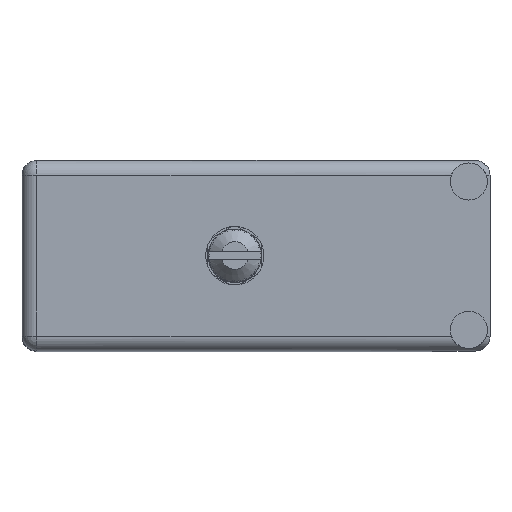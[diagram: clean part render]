
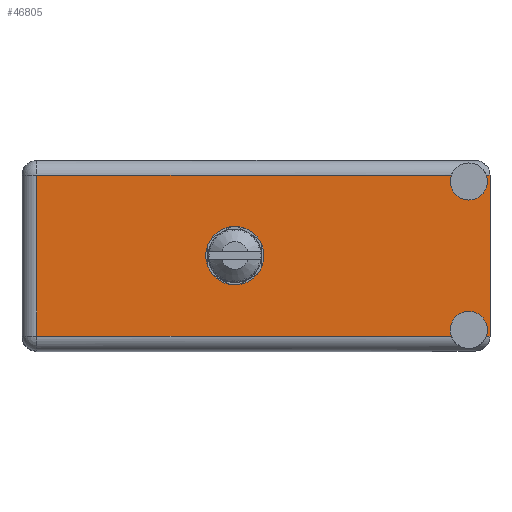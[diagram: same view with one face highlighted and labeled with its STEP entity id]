
A CAD part, top view. The second image highlights one B-rep face of the part: STEP entity #46805.
In plain terms, the highlighted face is planar.
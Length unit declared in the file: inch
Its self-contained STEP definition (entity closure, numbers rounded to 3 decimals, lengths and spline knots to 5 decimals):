
#217 = EDGE_CURVE ( 'NONE', #81219, #66211, #25588, .T. ) ;
#3424 = CARTESIAN_POINT ( 'NONE',  ( 2.19038, 1.566, -0.829 ) ) ;
#3814 = DIRECTION ( 'NONE',  ( 0., 1., 0. ) ) ;
#3861 = LINE ( 'NONE', #11633, #55414 ) ;
#5197 = CARTESIAN_POINT ( 'NONE',  ( 2.108, 1.566, -0.7995 ) ) ;
#6109 = CARTESIAN_POINT ( 'NONE',  ( 2.108, 1.566, -0.0995 ) ) ;
#7385 = AXIS2_PLACEMENT_3D ( 'NONE', #73167, #33031, #65398 ) ;
#7603 = VERTEX_POINT ( 'NONE', #69395 ) ;
#9852 = AXIS2_PLACEMENT_3D ( 'NONE', #26277, #73472, #17136 ) ;
#10412 = EDGE_CURVE ( 'NONE', #15194, #74606, #84376, .T. ) ;
#10895 = LINE ( 'NONE', #34693, #63753 ) ;
#11633 = CARTESIAN_POINT ( 'NONE',  ( 0., 1.566, -0.829 ) ) ;
#12533 = CARTESIAN_POINT ( 'NONE',  ( 0., 1.566, -0.829 ) ) ;
#14298 = CARTESIAN_POINT ( 'NONE',  ( 0.07, 1.566, -0.07 ) ) ;
#14692 = DIRECTION ( 'NONE',  ( 1., 0., 0. ) ) ;
#14764 = VERTEX_POINT ( 'NONE', #14298 ) ;
#15009 = ORIENTED_EDGE ( 'NONE', *, *, #86410, .T. ) ;
#15194 = VERTEX_POINT ( 'NONE', #44360 ) ;
#17136 = DIRECTION ( 'NONE',  ( 0., 0., 1. ) ) ;
#19042 = VERTEX_POINT ( 'NONE', #3424 ) ;
#19838 = CIRCLE ( 'NONE', #90225, 0.1375 ) ;
#21154 = CARTESIAN_POINT ( 'NONE',  ( 2.108, 1.566, -0.7995 ) ) ;
#21436 = DIRECTION ( 'NONE',  ( 0., 1., 0. ) ) ;
#25588 = CIRCLE ( 'NONE', #9852, 0.0875 ) ;
#26114 = CARTESIAN_POINT ( 'NONE',  ( 2.208, 1.566, -0.829 ) ) ;
#26277 = CARTESIAN_POINT ( 'NONE',  ( 2.108, 1.566, -0.0995 ) ) ;
#26294 = EDGE_CURVE ( 'NONE', #74606, #19042, #34455, .T. ) ;
#27013 = VERTEX_POINT ( 'NONE', #93159 ) ;
#27105 = VECTOR ( 'NONE', #92907, 39.37008 ) ;
#27858 = CARTESIAN_POINT ( 'NONE',  ( 2.208, 1.566, -0.07 ) ) ;
#28291 = FACE_OUTER_BOUND ( 'NONE', #92703, .T. ) ;
#30635 = ORIENTED_EDGE ( 'NONE', *, *, #26294, .F. ) ;
#30980 = ORIENTED_EDGE ( 'NONE', *, *, #10412, .F. ) ;
#32038 = CARTESIAN_POINT ( 'NONE',  ( 2.108, 1.566, -0.712 ) ) ;
#32820 = VERTEX_POINT ( 'NONE', #100616 ) ;
#33031 = DIRECTION ( 'NONE',  ( 0., 1., 0. ) ) ;
#34455 = CIRCLE ( 'NONE', #42797, 0.0875 ) ;
#34622 = EDGE_CURVE ( 'NONE', #89376, #19042, #49492, .T. ) ;
#34693 = CARTESIAN_POINT ( 'NONE',  ( 2.208, 1.566, -0.07 ) ) ;
#35151 = ORIENTED_EDGE ( 'NONE', *, *, #94289, .F. ) ;
#38454 = DIRECTION ( 'NONE',  ( 0., 0., 1. ) ) ;
#38522 = EDGE_CURVE ( 'NONE', #15194, #32820, #3861, .T. ) ;
#40767 = PLANE ( 'NONE',  #7385 ) ;
#42797 = AXIS2_PLACEMENT_3D ( 'NONE', #21154, #70147, #102629 ) ;
#43233 = CARTESIAN_POINT ( 'NONE',  ( 2.19038, 1.566, -0.07 ) ) ;
#44360 = CARTESIAN_POINT ( 'NONE',  ( 2.02562, 1.566, -0.829 ) ) ;
#44672 = LINE ( 'NONE', #67848, #27105 ) ;
#46805 = ADVANCED_FACE ( 'NONE', ( #49663, #28291 ), #40767, .T. ) ;
#46841 = DIRECTION ( 'NONE',  ( 0., 1., 0. ) ) ;
#48453 = CARTESIAN_POINT ( 'NONE',  ( 1.004, 1.566, -0.4495 ) ) ;
#49492 = LINE ( 'NONE', #12533, #100075 ) ;
#49663 = FACE_BOUND ( 'NONE', #64952, .T. ) ;
#52267 = VECTOR ( 'NONE', #89574, 39.37008 ) ;
#52943 = ORIENTED_EDGE ( 'NONE', *, *, #34622, .T. ) ;
#55414 = VECTOR ( 'NONE', #76007, 39.37008 ) ;
#55981 = VERTEX_POINT ( 'NONE', #102552 ) ;
#56037 = VECTOR ( 'NONE', #14692, 39.37008 ) ;
#56750 = CIRCLE ( 'NONE', #77811, 0.1375 ) ;
#56894 = VERTEX_POINT ( 'NONE', #27858 ) ;
#57766 = DIRECTION ( 'NONE',  ( 0., 0., 1. ) ) ;
#57842 = CARTESIAN_POINT ( 'NONE',  ( 0.07, 1.566, -0.899 ) ) ;
#60397 = EDGE_CURVE ( 'NONE', #27013, #55981, #19838, .T. ) ;
#60688 = DIRECTION ( 'NONE',  ( 1., 0., 0. ) ) ;
#61539 = EDGE_CURVE ( 'NONE', #14764, #7603, #10895, .T. ) ;
#62945 = DIRECTION ( 'NONE',  ( 0., 1., 0. ) ) ;
#63589 = EDGE_CURVE ( 'NONE', #32820, #14764, #92528, .T. ) ;
#63753 = VECTOR ( 'NONE', #60688, 39.37008 ) ;
#64362 = AXIS2_PLACEMENT_3D ( 'NONE', #5197, #3814, #68515 ) ;
#64952 = EDGE_LOOP ( 'NONE', ( #69880, #70934 ) ) ;
#65398 = DIRECTION ( 'NONE',  ( 0., 0., 1. ) ) ;
#65416 = ORIENTED_EDGE ( 'NONE', *, *, #61539, .T. ) ;
#66211 = VERTEX_POINT ( 'NONE', #91229 ) ;
#67510 = ORIENTED_EDGE ( 'NONE', *, *, #38522, .T. ) ;
#67756 = AXIS2_PLACEMENT_3D ( 'NONE', #6109, #46841, #38454 ) ;
#67848 = CARTESIAN_POINT ( 'NONE',  ( 2.208, 1.566, 0. ) ) ;
#68515 = DIRECTION ( 'NONE',  ( 0., 0., 1. ) ) ;
#69395 = CARTESIAN_POINT ( 'NONE',  ( 2.02562, 1.566, -0.07 ) ) ;
#69880 = ORIENTED_EDGE ( 'NONE', *, *, #79837, .F. ) ;
#70147 = DIRECTION ( 'NONE',  ( 0., 1., 0. ) ) ;
#70934 = ORIENTED_EDGE ( 'NONE', *, *, #60397, .F. ) ;
#72233 = CIRCLE ( 'NONE', #67756, 0.0875 ) ;
#73167 = CARTESIAN_POINT ( 'NONE',  ( 0., 1.566, -0.899 ) ) ;
#73472 = DIRECTION ( 'NONE',  ( 0., 1., 0. ) ) ;
#74606 = VERTEX_POINT ( 'NONE', #32038 ) ;
#76007 = DIRECTION ( 'NONE',  ( -1., 0., 0. ) ) ;
#76616 = DIRECTION ( 'NONE',  ( -1., 0., 0. ) ) ;
#77738 = ORIENTED_EDGE ( 'NONE', *, *, #96961, .F. ) ;
#77811 = AXIS2_PLACEMENT_3D ( 'NONE', #102186, #21436, #79258 ) ;
#79258 = DIRECTION ( 'NONE',  ( 0., 0., 1. ) ) ;
#79837 = EDGE_CURVE ( 'NONE', #55981, #27013, #56750, .T. ) ;
#81219 = VERTEX_POINT ( 'NONE', #43233 ) ;
#84376 = CIRCLE ( 'NONE', #64362, 0.0875 ) ;
#86410 = EDGE_CURVE ( 'NONE', #81219, #56894, #95188, .T. ) ;
#89376 = VERTEX_POINT ( 'NONE', #26114 ) ;
#89574 = DIRECTION ( 'NONE',  ( 0., 0., 1. ) ) ;
#90225 = AXIS2_PLACEMENT_3D ( 'NONE', #48453, #62945, #57766 ) ;
#90987 = ORIENTED_EDGE ( 'NONE', *, *, #63589, .T. ) ;
#91229 = CARTESIAN_POINT ( 'NONE',  ( 2.108, 1.566, -0.187 ) ) ;
#92528 = LINE ( 'NONE', #57842, #52267 ) ;
#92703 = EDGE_LOOP ( 'NONE', ( #65416, #35151, #94026, #15009, #77738, #52943, #30635, #30980, #67510, #90987 ) ) ;
#92907 = DIRECTION ( 'NONE',  ( 0., 0., 1. ) ) ;
#93159 = CARTESIAN_POINT ( 'NONE',  ( 1.004, 1.566, -0.587 ) ) ;
#94026 = ORIENTED_EDGE ( 'NONE', *, *, #217, .F. ) ;
#94289 = EDGE_CURVE ( 'NONE', #66211, #7603, #72233, .T. ) ;
#95188 = LINE ( 'NONE', #95370, #56037 ) ;
#95370 = CARTESIAN_POINT ( 'NONE',  ( 2.208, 1.566, -0.07 ) ) ;
#96961 = EDGE_CURVE ( 'NONE', #89376, #56894, #44672, .T. ) ;
#100075 = VECTOR ( 'NONE', #76616, 39.37008 ) ;
#100616 = CARTESIAN_POINT ( 'NONE',  ( 0.07, 1.566, -0.829 ) ) ;
#102186 = CARTESIAN_POINT ( 'NONE',  ( 1.004, 1.566, -0.4495 ) ) ;
#102552 = CARTESIAN_POINT ( 'NONE',  ( 1.004, 1.566, -0.312 ) ) ;
#102629 = DIRECTION ( 'NONE',  ( 0., 0., 1. ) ) ;
